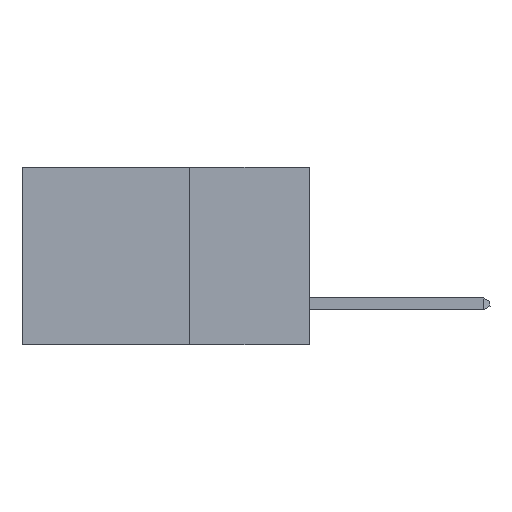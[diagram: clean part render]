
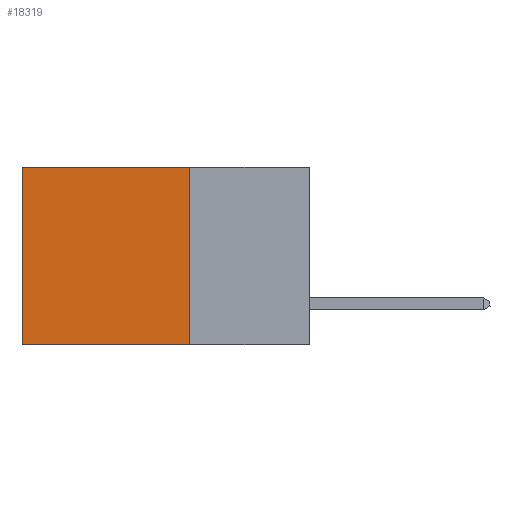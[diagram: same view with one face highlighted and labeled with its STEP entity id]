
A CAD part, left-side view. The second image highlights one B-rep face of the part: STEP entity #18319.
In plain terms, the highlighted planar face has unit normal (-1, 0, 0).
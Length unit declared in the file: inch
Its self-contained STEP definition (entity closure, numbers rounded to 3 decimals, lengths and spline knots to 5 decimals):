
#566 = VERTEX_POINT ( 'NONE', #8413 ) ;
#2236 = FACE_OUTER_BOUND ( 'NONE', #13105, .T. ) ;
#2735 = ORIENTED_EDGE ( 'NONE', *, *, #8180, .T. ) ;
#2791 = EDGE_CURVE ( 'NONE', #26271, #19369, #20006, .T. ) ;
#3379 = VECTOR ( 'NONE', #27031, 39.37008 ) ;
#3454 = ORIENTED_EDGE ( 'NONE', *, *, #2791, .F. ) ;
#3898 = DIRECTION ( 'NONE',  ( 1., 0., 0. ) ) ;
#5728 = ORIENTED_EDGE ( 'NONE', *, *, #16719, .F. ) ;
#5953 = LINE ( 'NONE', #13391, #22748 ) ;
#7872 = CARTESIAN_POINT ( 'NONE',  ( 0.2875, 0.6, -0.37 ) ) ;
#8180 = EDGE_CURVE ( 'NONE', #13167, #566, #5953, .T. ) ;
#8222 = VECTOR ( 'NONE', #16972, 39.37008 ) ;
#8349 = CARTESIAN_POINT ( 'NONE',  ( 0.2875, 0.25, 0. ) ) ;
#8413 = CARTESIAN_POINT ( 'NONE',  ( 0.2875, 0.6, 0. ) ) ;
#8519 = VECTOR ( 'NONE', #21636, 39.37008 ) ;
#8650 = ORIENTED_EDGE ( 'NONE', *, *, #16311, .T. ) ;
#13105 = EDGE_LOOP ( 'NONE', ( #8650, #3454, #5728, #2735 ) ) ;
#13167 = VERTEX_POINT ( 'NONE', #16214 ) ;
#13391 = CARTESIAN_POINT ( 'NONE',  ( 0.2875, 0.25, 0. ) ) ;
#15510 = DIRECTION ( 'NONE',  ( 0., 1., 0. ) ) ;
#16214 = CARTESIAN_POINT ( 'NONE',  ( 0.2875, 0.25, 0. ) ) ;
#16311 = EDGE_CURVE ( 'NONE', #566, #19369, #25167, .T. ) ;
#16688 = CARTESIAN_POINT ( 'NONE',  ( 0.2875, 0.25, 0. ) ) ;
#16702 = CARTESIAN_POINT ( 'NONE',  ( 0.2875, 0.25, -0.37 ) ) ;
#16719 = EDGE_CURVE ( 'NONE', #13167, #26271, #19629, .T. ) ;
#16972 = DIRECTION ( 'NONE',  ( 0., 1., 0. ) ) ;
#18319 = ADVANCED_FACE ( 'NONE', ( #2236 ), #26969, .F. ) ;
#18774 = DIRECTION ( 'NONE',  ( 0., 0., -1. ) ) ;
#19369 = VERTEX_POINT ( 'NONE', #7872 ) ;
#19541 = CARTESIAN_POINT ( 'NONE',  ( 0.2875, 0.6, 0. ) ) ;
#19629 = LINE ( 'NONE', #8349, #3379 ) ;
#20006 = LINE ( 'NONE', #16702, #8222 ) ;
#21636 = DIRECTION ( 'NONE',  ( 0., 0., -1. ) ) ;
#22466 = AXIS2_PLACEMENT_3D ( 'NONE', #16688, #3898, #18774 ) ;
#22748 = VECTOR ( 'NONE', #15510, 39.37008 ) ;
#24502 = CARTESIAN_POINT ( 'NONE',  ( 0.2875, 0.25, -0.37 ) ) ;
#25167 = LINE ( 'NONE', #19541, #8519 ) ;
#26271 = VERTEX_POINT ( 'NONE', #24502 ) ;
#26969 = PLANE ( 'NONE',  #22466 ) ;
#27031 = DIRECTION ( 'NONE',  ( 0., 0., -1. ) ) ;
